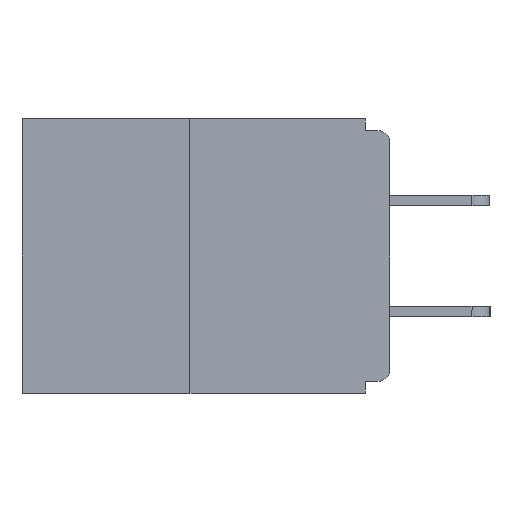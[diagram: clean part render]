
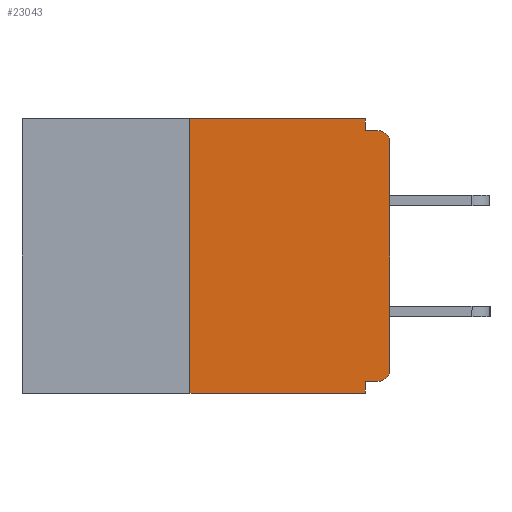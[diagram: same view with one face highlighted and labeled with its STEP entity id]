
A CAD part, left-side view. The second image highlights one B-rep face of the part: STEP entity #23043.
In plain terms, the highlighted planar face has unit normal (-1, 0, 0).
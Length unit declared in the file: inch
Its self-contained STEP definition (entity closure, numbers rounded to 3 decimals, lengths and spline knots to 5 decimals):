
#267 = CARTESIAN_POINT ( 'NONE',  ( 0., 0.46, 0. ) ) ;
#281 = VECTOR ( 'NONE', #16693, 39.37008 ) ;
#463 = ORIENTED_EDGE ( 'NONE', *, *, #20277, .F. ) ;
#1451 = VERTEX_POINT ( 'NONE', #9494 ) ;
#1679 = LINE ( 'NONE', #24922, #24987 ) ;
#2041 = CIRCLE ( 'NONE', #21426, 0.015 ) ;
#2290 = ORIENTED_EDGE ( 'NONE', *, *, #25418, .F. ) ;
#2625 = DIRECTION ( 'NONE',  ( 0., 0., -1. ) ) ;
#3453 = DIRECTION ( 'NONE',  ( 0., 0., -1. ) ) ;
#3592 = LINE ( 'NONE', #13138, #14870 ) ;
#3628 = DIRECTION ( 'NONE',  ( 0., -1., 0. ) ) ;
#4099 = VERTEX_POINT ( 'NONE', #21810 ) ;
#4206 = CARTESIAN_POINT ( 'NONE',  ( 0., 0.25, -0.343 ) ) ;
#4271 = DIRECTION ( 'NONE',  ( 0., -1., 0. ) ) ;
#4419 = EDGE_CURVE ( 'NONE', #21502, #11855, #10706, .T. ) ;
#4426 = LINE ( 'NONE', #16154, #27690 ) ;
#4546 = VECTOR ( 'NONE', #3453, 39.37008 ) ;
#4869 = AXIS2_PLACEMENT_3D ( 'NONE', #27590, #27398, #9516 ) ;
#5871 = ORIENTED_EDGE ( 'NONE', *, *, #26539, .F. ) ;
#7311 = CARTESIAN_POINT ( 'NONE',  ( 0., 0.25, 0. ) ) ;
#8007 = CARTESIAN_POINT ( 'NONE',  ( 0., 0.031, 0. ) ) ;
#8776 = EDGE_CURVE ( 'NONE', #11162, #4099, #1679, .T. ) ;
#8847 = ORIENTED_EDGE ( 'NONE', *, *, #21107, .T. ) ;
#9011 = LINE ( 'NONE', #26852, #20200 ) ;
#9396 = LINE ( 'NONE', #267, #26289 ) ;
#9494 = CARTESIAN_POINT ( 'NONE',  ( 0., 0.031, 0. ) ) ;
#9516 = DIRECTION ( 'NONE',  ( 0., 0., -1. ) ) ;
#9584 = VERTEX_POINT ( 'NONE', #12317 ) ;
#9719 = ORIENTED_EDGE ( 'NONE', *, *, #16214, .T. ) ;
#9897 = CARTESIAN_POINT ( 'NONE',  ( 0., 0., -0.328 ) ) ;
#10706 = LINE ( 'NONE', #9897, #18397 ) ;
#10884 = EDGE_CURVE ( 'NONE', #29205, #9584, #9011, .T. ) ;
#10914 = CARTESIAN_POINT ( 'NONE',  ( 0., 0.015, -0.03 ) ) ;
#11162 = VERTEX_POINT ( 'NONE', #21086 ) ;
#11823 = PLANE ( 'NONE',  #4869 ) ;
#11855 = VERTEX_POINT ( 'NONE', #28891 ) ;
#12153 = ORIENTED_EDGE ( 'NONE', *, *, #10884, .T. ) ;
#12317 = CARTESIAN_POINT ( 'NONE',  ( 0., 0., -0.03 ) ) ;
#12515 = EDGE_CURVE ( 'NONE', #28400, #19039, #19289, .T. ) ;
#13138 = CARTESIAN_POINT ( 'NONE',  ( 0., 0.46, -0.343 ) ) ;
#14712 = VERTEX_POINT ( 'NONE', #19467 ) ;
#14811 = CARTESIAN_POINT ( 'NONE',  ( 0., 0.015, -0.328 ) ) ;
#14870 = VECTOR ( 'NONE', #4271, 39.37008 ) ;
#16154 = CARTESIAN_POINT ( 'NONE',  ( 0., 0.031, -0.343 ) ) ;
#16214 = EDGE_CURVE ( 'NONE', #28400, #14712, #3592, .T. ) ;
#16684 = EDGE_LOOP ( 'NONE', ( #5871, #28285, #9719, #2290, #26763, #26992, #12153, #8847, #21815, #463 ) ) ;
#16693 = DIRECTION ( 'NONE',  ( 0., 0., 1. ) ) ;
#16788 = CARTESIAN_POINT ( 'NONE',  ( 0., 0.25, 0. ) ) ;
#16910 = AXIS2_PLACEMENT_3D ( 'NONE', #10914, #26664, #28943 ) ;
#17328 = DIRECTION ( 'NONE',  ( -1., 0., 0. ) ) ;
#18105 = CARTESIAN_POINT ( 'NONE',  ( 0., 0., -0.313 ) ) ;
#18397 = VECTOR ( 'NONE', #21173, 39.37008 ) ;
#19039 = VERTEX_POINT ( 'NONE', #7311 ) ;
#19289 = LINE ( 'NONE', #16788, #281 ) ;
#19467 = CARTESIAN_POINT ( 'NONE',  ( 0., 0.031, -0.343 ) ) ;
#20200 = VECTOR ( 'NONE', #22520, 39.37008 ) ;
#20277 = EDGE_CURVE ( 'NONE', #1451, #11162, #26743, .T. ) ;
#20425 = DIRECTION ( 'NONE',  ( 0., -1., 0. ) ) ;
#20533 = FACE_OUTER_BOUND ( 'NONE', #16684, .T. ) ;
#20663 = EDGE_CURVE ( 'NONE', #21502, #29205, #2041, .T. ) ;
#21086 = CARTESIAN_POINT ( 'NONE',  ( 0., 0.031, -0.015 ) ) ;
#21107 = EDGE_CURVE ( 'NONE', #9584, #4099, #23866, .T. ) ;
#21173 = DIRECTION ( 'NONE',  ( 0., 1., 0. ) ) ;
#21426 = AXIS2_PLACEMENT_3D ( 'NONE', #26530, #17328, #26429 ) ;
#21502 = VERTEX_POINT ( 'NONE', #14811 ) ;
#21810 = CARTESIAN_POINT ( 'NONE',  ( 0., 0.015, -0.015 ) ) ;
#21815 = ORIENTED_EDGE ( 'NONE', *, *, #8776, .F. ) ;
#22520 = DIRECTION ( 'NONE',  ( 0., 0., 1. ) ) ;
#23043 = ADVANCED_FACE ( 'NONE', ( #20533 ), #11823, .F. ) ;
#23866 = CIRCLE ( 'NONE', #16910, 0.015 ) ;
#24922 = CARTESIAN_POINT ( 'NONE',  ( 0., 0., -0.015 ) ) ;
#24987 = VECTOR ( 'NONE', #20425, 39.37008 ) ;
#25418 = EDGE_CURVE ( 'NONE', #11855, #14712, #4426, .T. ) ;
#26289 = VECTOR ( 'NONE', #3628, 39.37008 ) ;
#26429 = DIRECTION ( 'NONE',  ( 0., 0., -1. ) ) ;
#26530 = CARTESIAN_POINT ( 'NONE',  ( 0., 0.015, -0.313 ) ) ;
#26539 = EDGE_CURVE ( 'NONE', #19039, #1451, #9396, .T. ) ;
#26664 = DIRECTION ( 'NONE',  ( -1., 0., 0. ) ) ;
#26743 = LINE ( 'NONE', #8007, #4546 ) ;
#26763 = ORIENTED_EDGE ( 'NONE', *, *, #4419, .F. ) ;
#26852 = CARTESIAN_POINT ( 'NONE',  ( 0., 0., 0. ) ) ;
#26992 = ORIENTED_EDGE ( 'NONE', *, *, #20663, .T. ) ;
#27398 = DIRECTION ( 'NONE',  ( 1., 0., 0. ) ) ;
#27590 = CARTESIAN_POINT ( 'NONE',  ( 0., 0.46, 0. ) ) ;
#27690 = VECTOR ( 'NONE', #2625, 39.37008 ) ;
#28285 = ORIENTED_EDGE ( 'NONE', *, *, #12515, .F. ) ;
#28400 = VERTEX_POINT ( 'NONE', #4206 ) ;
#28891 = CARTESIAN_POINT ( 'NONE',  ( 0., 0.031, -0.328 ) ) ;
#28943 = DIRECTION ( 'NONE',  ( 0., 0., -1. ) ) ;
#29205 = VERTEX_POINT ( 'NONE', #18105 ) ;
